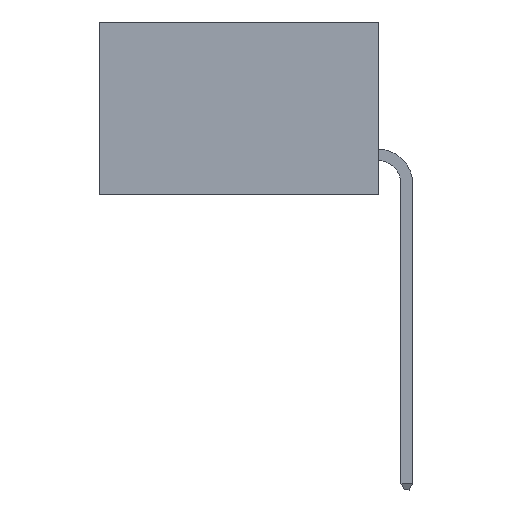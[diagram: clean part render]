
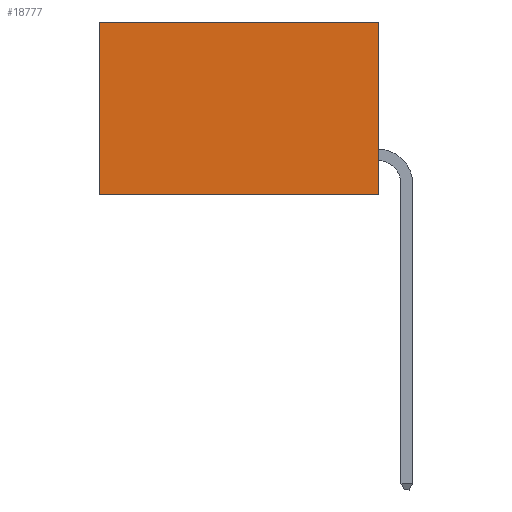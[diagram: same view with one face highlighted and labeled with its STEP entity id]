
A CAD part, left-side view. The second image highlights one B-rep face of the part: STEP entity #18777.
In plain terms, the highlighted planar face has unit normal (-1, 0, 0).
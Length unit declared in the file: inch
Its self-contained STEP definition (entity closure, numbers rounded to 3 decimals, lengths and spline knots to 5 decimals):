
#153 = PLANE ( 'NONE',  #11485 ) ;
#338 = ORIENTED_EDGE ( 'NONE', *, *, #2251, .T. ) ;
#1729 = DIRECTION ( 'NONE',  ( 0., 1., 0. ) ) ;
#2251 = EDGE_CURVE ( 'NONE', #18714, #4732, #12394, .T. ) ;
#3221 = ORIENTED_EDGE ( 'NONE', *, *, #18593, .F. ) ;
#3350 = EDGE_LOOP ( 'NONE', ( #338, #3221, #16619, #18677 ) ) ;
#3884 = VERTEX_POINT ( 'NONE', #17253 ) ;
#4732 = VERTEX_POINT ( 'NONE', #19581 ) ;
#5087 = LINE ( 'NONE', #8846, #12595 ) ;
#5343 = VECTOR ( 'NONE', #12048, 39.37008 ) ;
#5932 = EDGE_CURVE ( 'NONE', #17019, #3884, #5087, .T. ) ;
#6262 = DIRECTION ( 'NONE',  ( 1., 0., 0. ) ) ;
#7014 = VECTOR ( 'NONE', #16090, 39.37008 ) ;
#8846 = CARTESIAN_POINT ( 'NONE',  ( 0.298, 0., 0. ) ) ;
#10779 = CARTESIAN_POINT ( 'NONE',  ( 0.298, 0., 0. ) ) ;
#10820 = DIRECTION ( 'NONE',  ( 0., 0., -1. ) ) ;
#10901 = CARTESIAN_POINT ( 'NONE',  ( 0.298, 0., 0. ) ) ;
#11485 = AXIS2_PLACEMENT_3D ( 'NONE', #10901, #6262, #18696 ) ;
#11596 = EDGE_CURVE ( 'NONE', #17019, #18714, #11780, .T. ) ;
#11780 = LINE ( 'NONE', #10779, #15390 ) ;
#11916 = CARTESIAN_POINT ( 'NONE',  ( 0.298, 0.6, 0. ) ) ;
#12048 = DIRECTION ( 'NONE',  ( 0., 0., -1. ) ) ;
#12394 = LINE ( 'NONE', #11916, #5343 ) ;
#12595 = VECTOR ( 'NONE', #10820, 39.37008 ) ;
#14033 = CARTESIAN_POINT ( 'NONE',  ( 0.298, 0., 0. ) ) ;
#15390 = VECTOR ( 'NONE', #1729, 39.37008 ) ;
#16032 = CARTESIAN_POINT ( 'NONE',  ( 0.298, 0., -0.37 ) ) ;
#16090 = DIRECTION ( 'NONE',  ( 0., 1., 0. ) ) ;
#16452 = LINE ( 'NONE', #16032, #7014 ) ;
#16619 = ORIENTED_EDGE ( 'NONE', *, *, #5932, .F. ) ;
#17019 = VERTEX_POINT ( 'NONE', #14033 ) ;
#17253 = CARTESIAN_POINT ( 'NONE',  ( 0.298, 0., -0.37 ) ) ;
#18082 = CARTESIAN_POINT ( 'NONE',  ( 0.298, 0.6, 0. ) ) ;
#18593 = EDGE_CURVE ( 'NONE', #3884, #4732, #16452, .T. ) ;
#18677 = ORIENTED_EDGE ( 'NONE', *, *, #11596, .T. ) ;
#18696 = DIRECTION ( 'NONE',  ( 0., 0., -1. ) ) ;
#18714 = VERTEX_POINT ( 'NONE', #18082 ) ;
#18777 = ADVANCED_FACE ( 'NONE', ( #19099 ), #153, .F. ) ;
#19099 = FACE_OUTER_BOUND ( 'NONE', #3350, .T. ) ;
#19581 = CARTESIAN_POINT ( 'NONE',  ( 0.298, 0.6, -0.37 ) ) ;
